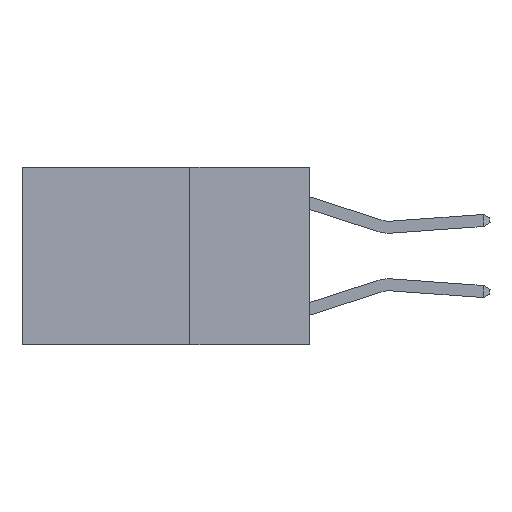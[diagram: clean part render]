
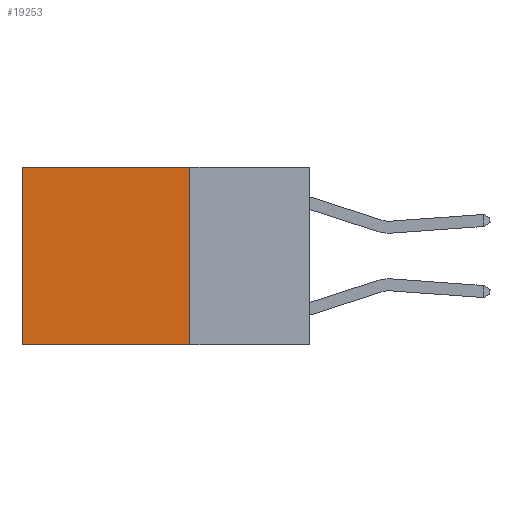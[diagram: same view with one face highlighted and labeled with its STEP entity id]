
A CAD part, left-side view. The second image highlights one B-rep face of the part: STEP entity #19253.
In plain terms, the highlighted planar face has unit normal (-1, 0, 0).
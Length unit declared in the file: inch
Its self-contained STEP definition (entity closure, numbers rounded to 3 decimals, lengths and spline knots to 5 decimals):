
#24 = VERTEX_POINT ( 'NONE', #5027 ) ;
#632 = DIRECTION ( 'NONE',  ( 0., 1., 0. ) ) ;
#757 = ORIENTED_EDGE ( 'NONE', *, *, #22408, .T. ) ;
#1146 = DIRECTION ( 'NONE',  ( 0., 0., -1. ) ) ;
#1203 = EDGE_LOOP ( 'NONE', ( #757, #9920, #10940, #10312 ) ) ;
#1947 = VERTEX_POINT ( 'NONE', #5338 ) ;
#4926 = CARTESIAN_POINT ( 'NONE',  ( 0.2625, 0.25, 0. ) ) ;
#5027 = CARTESIAN_POINT ( 'NONE',  ( 0.2625, 0.6, 0. ) ) ;
#5338 = CARTESIAN_POINT ( 'NONE',  ( 0.2625, 0.25, -0.37 ) ) ;
#6737 = EDGE_CURVE ( 'NONE', #20376, #24, #21087, .T. ) ;
#7976 = LINE ( 'NONE', #11615, #14760 ) ;
#8263 = PLANE ( 'NONE',  #14726 ) ;
#8620 = DIRECTION ( 'NONE',  ( 1., 0., 0. ) ) ;
#8951 = VECTOR ( 'NONE', #15907, 39.37008 ) ;
#9377 = CARTESIAN_POINT ( 'NONE',  ( 0.2625, 0.6, 0. ) ) ;
#9557 = LINE ( 'NONE', #14876, #18570 ) ;
#9920 = ORIENTED_EDGE ( 'NONE', *, *, #21922, .F. ) ;
#10259 = FACE_OUTER_BOUND ( 'NONE', #1203, .T. ) ;
#10312 = ORIENTED_EDGE ( 'NONE', *, *, #6737, .T. ) ;
#10940 = ORIENTED_EDGE ( 'NONE', *, *, #17737, .F. ) ;
#11615 = CARTESIAN_POINT ( 'NONE',  ( 0.2625, 0.25, -0.37 ) ) ;
#11753 = VECTOR ( 'NONE', #13142, 39.37008 ) ;
#13142 = DIRECTION ( 'NONE',  ( 0., 0., -1. ) ) ;
#13257 = LINE ( 'NONE', #9377, #11753 ) ;
#13920 = CARTESIAN_POINT ( 'NONE',  ( 0.2625, 0.25, 0. ) ) ;
#13925 = CARTESIAN_POINT ( 'NONE',  ( 0.2625, 0.25, 0. ) ) ;
#14726 = AXIS2_PLACEMENT_3D ( 'NONE', #13925, #8620, #1146 ) ;
#14760 = VECTOR ( 'NONE', #632, 39.37008 ) ;
#14876 = CARTESIAN_POINT ( 'NONE',  ( 0.2625, 0.25, 0. ) ) ;
#14942 = CARTESIAN_POINT ( 'NONE',  ( 0.2625, 0.6, -0.37 ) ) ;
#15907 = DIRECTION ( 'NONE',  ( 0., 1., 0. ) ) ;
#16968 = DIRECTION ( 'NONE',  ( 0., 0., -1. ) ) ;
#17737 = EDGE_CURVE ( 'NONE', #20376, #1947, #9557, .T. ) ;
#18570 = VECTOR ( 'NONE', #16968, 39.37008 ) ;
#19253 = ADVANCED_FACE ( 'NONE', ( #10259 ), #8263, .F. ) ;
#20376 = VERTEX_POINT ( 'NONE', #4926 ) ;
#20714 = VERTEX_POINT ( 'NONE', #14942 ) ;
#21087 = LINE ( 'NONE', #13920, #8951 ) ;
#21922 = EDGE_CURVE ( 'NONE', #1947, #20714, #7976, .T. ) ;
#22408 = EDGE_CURVE ( 'NONE', #24, #20714, #13257, .T. ) ;
